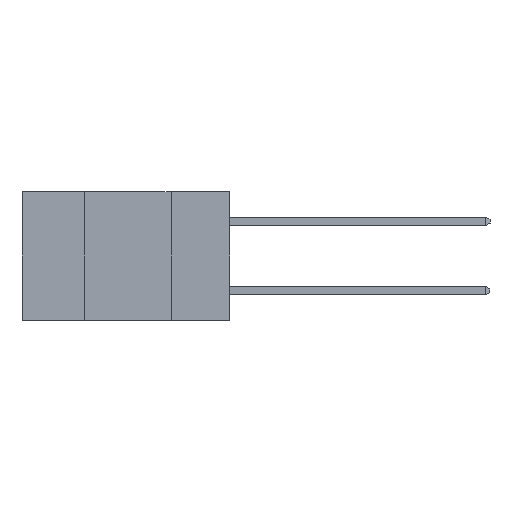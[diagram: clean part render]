
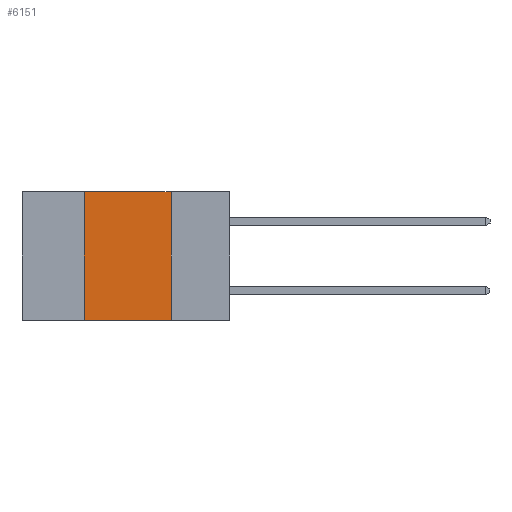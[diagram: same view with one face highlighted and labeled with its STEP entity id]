
A CAD part, left-side view. The second image highlights one B-rep face of the part: STEP entity #6151.
In plain terms, the highlighted planar face has unit normal (-1, 0, 0).
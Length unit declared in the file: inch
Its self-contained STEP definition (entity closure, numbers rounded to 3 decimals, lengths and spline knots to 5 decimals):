
#1017 = VERTEX_POINT ( 'NONE', #2223 ) ;
#1452 = CARTESIAN_POINT ( 'NONE',  ( 0., 0.17, 0. ) ) ;
#1769 = VERTEX_POINT ( 'NONE', #7352 ) ;
#2042 = LINE ( 'NONE', #13193, #4678 ) ;
#2077 = AXIS2_PLACEMENT_3D ( 'NONE', #13515, #13575, #7349 ) ;
#2223 = CARTESIAN_POINT ( 'NONE',  ( 0., 0.17, -0.37 ) ) ;
#2949 = CARTESIAN_POINT ( 'NONE',  ( 0., 0.17, 0. ) ) ;
#3835 = VECTOR ( 'NONE', #5705, 39.37008 ) ;
#4025 = CARTESIAN_POINT ( 'NONE',  ( 0., 0.42, 0. ) ) ;
#4045 = ORIENTED_EDGE ( 'NONE', *, *, #9553, .F. ) ;
#4678 = VECTOR ( 'NONE', #13814, 39.37008 ) ;
#5094 = PLANE ( 'NONE',  #2077 ) ;
#5639 = EDGE_CURVE ( 'NONE', #6879, #1017, #12813, .T. ) ;
#5653 = VERTEX_POINT ( 'NONE', #4025 ) ;
#5705 = DIRECTION ( 'NONE',  ( 0., 0., -1. ) ) ;
#6151 = ADVANCED_FACE ( 'NONE', ( #8801 ), #5094, .F. ) ;
#6449 = ORIENTED_EDGE ( 'NONE', *, *, #11077, .F. ) ;
#6879 = VERTEX_POINT ( 'NONE', #2949 ) ;
#7349 = DIRECTION ( 'NONE',  ( 0., 0., -1. ) ) ;
#7352 = CARTESIAN_POINT ( 'NONE',  ( 0., 0.42, -0.37 ) ) ;
#8801 = FACE_OUTER_BOUND ( 'NONE', #11459, .T. ) ;
#9553 = EDGE_CURVE ( 'NONE', #1769, #5653, #2042, .T. ) ;
#10544 = ORIENTED_EDGE ( 'NONE', *, *, #12400, .T. ) ;
#11077 = EDGE_CURVE ( 'NONE', #5653, #6879, #14449, .T. ) ;
#11232 = DIRECTION ( 'NONE',  ( 0., -1., 0. ) ) ;
#11360 = DIRECTION ( 'NONE',  ( 0., -1., 0. ) ) ;
#11459 = EDGE_LOOP ( 'NONE', ( #12009, #6449, #4045, #10544 ) ) ;
#11740 = VECTOR ( 'NONE', #11232, 39.37008 ) ;
#12009 = ORIENTED_EDGE ( 'NONE', *, *, #5639, .F. ) ;
#12195 = CARTESIAN_POINT ( 'NONE',  ( 0., 0.6, -0.37 ) ) ;
#12400 = EDGE_CURVE ( 'NONE', #1769, #1017, #14600, .T. ) ;
#12813 = LINE ( 'NONE', #1452, #3835 ) ;
#13193 = CARTESIAN_POINT ( 'NONE',  ( 0., 0.42, 0. ) ) ;
#13505 = CARTESIAN_POINT ( 'NONE',  ( 0., 0.6, 0. ) ) ;
#13515 = CARTESIAN_POINT ( 'NONE',  ( 0., 0.6, 0. ) ) ;
#13575 = DIRECTION ( 'NONE',  ( 1., 0., 0. ) ) ;
#13814 = DIRECTION ( 'NONE',  ( 0., 0., 1. ) ) ;
#14112 = VECTOR ( 'NONE', #11360, 39.37008 ) ;
#14449 = LINE ( 'NONE', #13505, #14112 ) ;
#14600 = LINE ( 'NONE', #12195, #11740 ) ;
